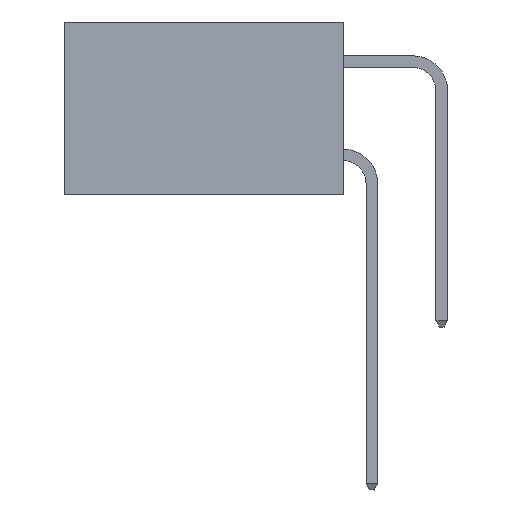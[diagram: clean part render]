
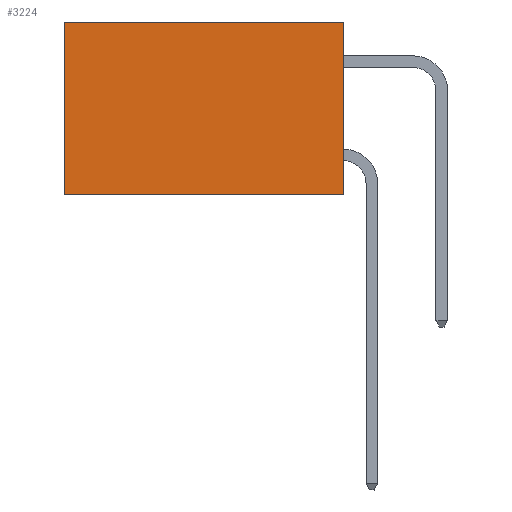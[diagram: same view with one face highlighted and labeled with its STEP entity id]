
A CAD part, left-side view. The second image highlights one B-rep face of the part: STEP entity #3224.
In plain terms, the highlighted planar face has unit normal (-1, 0, 0).
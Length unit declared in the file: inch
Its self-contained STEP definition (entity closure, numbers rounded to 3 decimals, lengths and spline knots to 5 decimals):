
#41 = EDGE_CURVE ( 'NONE', #7435, #591, #5710, .T. ) ;
#90 = ORIENTED_EDGE ( 'NONE', *, *, #5737, .T. ) ;
#485 = CARTESIAN_POINT ( 'NONE',  ( 0.2615, 0.6, -0.37 ) ) ;
#531 = CARTESIAN_POINT ( 'NONE',  ( 0.2615, 0., -0.37 ) ) ;
#546 = LINE ( 'NONE', #7967, #3229 ) ;
#591 = VERTEX_POINT ( 'NONE', #4893 ) ;
#663 = CARTESIAN_POINT ( 'NONE',  ( 0.2615, 0., 0. ) ) ;
#1049 = DIRECTION ( 'NONE',  ( 0., 0., -1. ) ) ;
#1366 = ORIENTED_EDGE ( 'NONE', *, *, #2807, .T. ) ;
#2005 = LINE ( 'NONE', #7629, #9258 ) ;
#2181 = VERTEX_POINT ( 'NONE', #10121 ) ;
#2372 = DIRECTION ( 'NONE',  ( 0., 0., -1. ) ) ;
#2508 = LINE ( 'NONE', #485, #8170 ) ;
#2807 = EDGE_CURVE ( 'NONE', #2181, #7556, #2508, .T. ) ;
#3224 = ADVANCED_FACE ( 'NONE', ( #7885 ), #4217, .F. ) ;
#3229 = VECTOR ( 'NONE', #3507, 39.37008 ) ;
#3507 = DIRECTION ( 'NONE',  ( 0., 1., 0. ) ) ;
#4217 = PLANE ( 'NONE',  #9912 ) ;
#4893 = CARTESIAN_POINT ( 'NONE',  ( 0.2615, 0., -0.37 ) ) ;
#5588 = VECTOR ( 'NONE', #1049, 39.37008 ) ;
#5710 = LINE ( 'NONE', #11278, #5588 ) ;
#5737 = EDGE_CURVE ( 'NONE', #7435, #2181, #2005, .T. ) ;
#6072 = DIRECTION ( 'NONE',  ( 0., 0., -1. ) ) ;
#6153 = EDGE_CURVE ( 'NONE', #591, #7556, #546, .T. ) ;
#6973 = DIRECTION ( 'NONE',  ( 1., 0., 0. ) ) ;
#7435 = VERTEX_POINT ( 'NONE', #663 ) ;
#7556 = VERTEX_POINT ( 'NONE', #9230 ) ;
#7629 = CARTESIAN_POINT ( 'NONE',  ( 0.2615, 0., 0. ) ) ;
#7885 = FACE_OUTER_BOUND ( 'NONE', #11594, .T. ) ;
#7967 = CARTESIAN_POINT ( 'NONE',  ( 0.2615, 0., -0.37 ) ) ;
#8170 = VECTOR ( 'NONE', #6072, 39.37008 ) ;
#9075 = DIRECTION ( 'NONE',  ( 0., 1., 0. ) ) ;
#9230 = CARTESIAN_POINT ( 'NONE',  ( 0.2615, 0.6, -0.37 ) ) ;
#9258 = VECTOR ( 'NONE', #9075, 39.37008 ) ;
#9631 = ORIENTED_EDGE ( 'NONE', *, *, #6153, .F. ) ;
#9912 = AXIS2_PLACEMENT_3D ( 'NONE', #531, #6973, #2372 ) ;
#10121 = CARTESIAN_POINT ( 'NONE',  ( 0.2615, 0.6, 0. ) ) ;
#11278 = CARTESIAN_POINT ( 'NONE',  ( 0.2615, 0., -0.37 ) ) ;
#11594 = EDGE_LOOP ( 'NONE', ( #1366, #9631, #11861, #90 ) ) ;
#11861 = ORIENTED_EDGE ( 'NONE', *, *, #41, .F. ) ;
